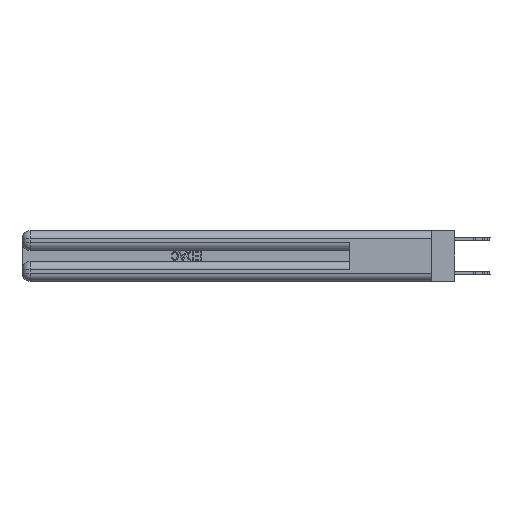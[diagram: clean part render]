
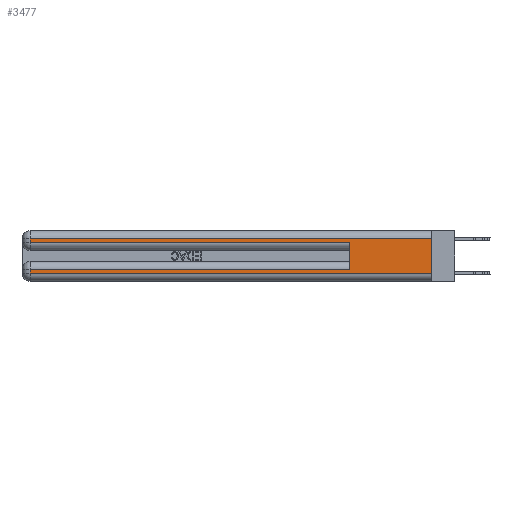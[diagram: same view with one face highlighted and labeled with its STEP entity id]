
A CAD part, left-side view. The second image highlights one B-rep face of the part: STEP entity #3477.
In plain terms, the highlighted planar face has unit normal (-1, 0, 0).
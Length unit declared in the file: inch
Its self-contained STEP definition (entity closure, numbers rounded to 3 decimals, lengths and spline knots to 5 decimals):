
#365 = EDGE_CURVE ( 'NONE', #21738, #10940, #8652, .T. ) ;
#840 = VECTOR ( 'NONE', #8835, 39.37008 ) ;
#2394 = DIRECTION ( 'NONE',  ( 0., 0., 1. ) ) ;
#2588 = DIRECTION ( 'NONE',  ( 0., -1., 0. ) ) ;
#3330 = VERTEX_POINT ( 'NONE', #28431 ) ;
#3477 = ADVANCED_FACE ( 'NONE', ( #18654 ), #32441, .F. ) ;
#3556 = CARTESIAN_POINT ( 'NONE',  ( 0., 0., 0.06 ) ) ;
#3560 = ORIENTED_EDGE ( 'NONE', *, *, #11188, .T. ) ;
#4733 = DIRECTION ( 'NONE',  ( 1., 0., 0. ) ) ;
#4814 = VECTOR ( 'NONE', #10204, 39.37008 ) ;
#5035 = LINE ( 'NONE', #16944, #18535 ) ;
#5293 = CARTESIAN_POINT ( 'NONE',  ( 0., 2.94, 0.285 ) ) ;
#6053 = EDGE_CURVE ( 'NONE', #16733, #24784, #5035, .T. ) ;
#6169 = CARTESIAN_POINT ( 'NONE',  ( 0., 0., 0.31 ) ) ;
#6559 = EDGE_CURVE ( 'NONE', #29969, #24213, #11971, .T. ) ;
#6900 = ORIENTED_EDGE ( 'NONE', *, *, #23633, .T. ) ;
#7769 = VECTOR ( 'NONE', #2588, 39.37008 ) ;
#8652 = LINE ( 'NONE', #22766, #840 ) ;
#8835 = DIRECTION ( 'NONE',  ( 0., -1., 0. ) ) ;
#10204 = DIRECTION ( 'NONE',  ( 0., 1., 0. ) ) ;
#10546 = DIRECTION ( 'NONE',  ( 0., 1., 0. ) ) ;
#10940 = VERTEX_POINT ( 'NONE', #21769 ) ;
#10949 = VECTOR ( 'NONE', #25359, 39.37008 ) ;
#11188 = EDGE_CURVE ( 'NONE', #29969, #3330, #15332, .T. ) ;
#11255 = VECTOR ( 'NONE', #2394, 39.37008 ) ;
#11971 = LINE ( 'NONE', #28286, #10949 ) ;
#12835 = ORIENTED_EDGE ( 'NONE', *, *, #26679, .T. ) ;
#13897 = DIRECTION ( 'NONE',  ( 0., 0., -1. ) ) ;
#14041 = EDGE_CURVE ( 'NONE', #16733, #10940, #27178, .T. ) ;
#14416 = VECTOR ( 'NONE', #18221, 39.37008 ) ;
#14580 = EDGE_LOOP ( 'NONE', ( #23254, #3560, #6900, #23610, #21224, #33195, #16332, #12835 ) ) ;
#15147 = CARTESIAN_POINT ( 'NONE',  ( 0., 0., 0.31 ) ) ;
#15332 = LINE ( 'NONE', #15147, #4814 ) ;
#15746 = CARTESIAN_POINT ( 'NONE',  ( 0., 0., 0.37 ) ) ;
#16116 = VERTEX_POINT ( 'NONE', #23806 ) ;
#16167 = CARTESIAN_POINT ( 'NONE',  ( 0., 0.6, 0.145 ) ) ;
#16332 = ORIENTED_EDGE ( 'NONE', *, *, #33027, .T. ) ;
#16733 = VERTEX_POINT ( 'NONE', #19499 ) ;
#16944 = CARTESIAN_POINT ( 'NONE',  ( 0., 0., 0.085 ) ) ;
#18221 = DIRECTION ( 'NONE',  ( 0., 0., -1. ) ) ;
#18535 = VECTOR ( 'NONE', #10546, 39.37008 ) ;
#18577 = LINE ( 'NONE', #29430, #14416 ) ;
#18654 = FACE_OUTER_BOUND ( 'NONE', #14580, .T. ) ;
#19499 = CARTESIAN_POINT ( 'NONE',  ( 0., 0.6, 0.085 ) ) ;
#21224 = ORIENTED_EDGE ( 'NONE', *, *, #14041, .F. ) ;
#21738 = VERTEX_POINT ( 'NONE', #5293 ) ;
#21769 = CARTESIAN_POINT ( 'NONE',  ( 0., 0.6, 0.285 ) ) ;
#22766 = CARTESIAN_POINT ( 'NONE',  ( 0., 0., 0.285 ) ) ;
#23254 = ORIENTED_EDGE ( 'NONE', *, *, #6559, .F. ) ;
#23610 = ORIENTED_EDGE ( 'NONE', *, *, #365, .T. ) ;
#23633 = EDGE_CURVE ( 'NONE', #3330, #21738, #25623, .T. ) ;
#23806 = CARTESIAN_POINT ( 'NONE',  ( 0., 2.94, 0.06 ) ) ;
#23835 = DIRECTION ( 'NONE',  ( 0., 0., -1. ) ) ;
#24213 = VERTEX_POINT ( 'NONE', #3556 ) ;
#24784 = VERTEX_POINT ( 'NONE', #27330 ) ;
#25359 = DIRECTION ( 'NONE',  ( 0., 0., -1. ) ) ;
#25623 = LINE ( 'NONE', #27832, #33446 ) ;
#26679 = EDGE_CURVE ( 'NONE', #16116, #24213, #36129, .T. ) ;
#26997 = CARTESIAN_POINT ( 'NONE',  ( 0., 0., 0.06 ) ) ;
#27178 = LINE ( 'NONE', #16167, #11255 ) ;
#27330 = CARTESIAN_POINT ( 'NONE',  ( 0., 2.94, 0.085 ) ) ;
#27832 = CARTESIAN_POINT ( 'NONE',  ( 0., 2.94, 0.37 ) ) ;
#28286 = CARTESIAN_POINT ( 'NONE',  ( 0., 0., 0.37 ) ) ;
#28431 = CARTESIAN_POINT ( 'NONE',  ( 0., 2.94, 0.31 ) ) ;
#29430 = CARTESIAN_POINT ( 'NONE',  ( 0., 2.94, 0.37 ) ) ;
#29969 = VERTEX_POINT ( 'NONE', #6169 ) ;
#32441 = PLANE ( 'NONE',  #34020 ) ;
#33027 = EDGE_CURVE ( 'NONE', #24784, #16116, #18577, .T. ) ;
#33195 = ORIENTED_EDGE ( 'NONE', *, *, #6053, .T. ) ;
#33446 = VECTOR ( 'NONE', #13897, 39.37008 ) ;
#34020 = AXIS2_PLACEMENT_3D ( 'NONE', #15746, #4733, #23835 ) ;
#36129 = LINE ( 'NONE', #26997, #7769 ) ;
